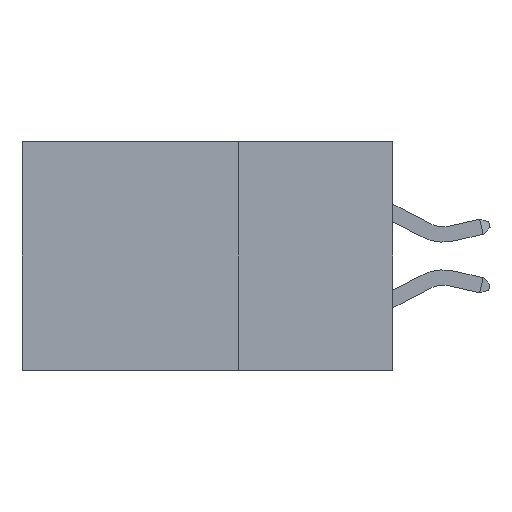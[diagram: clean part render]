
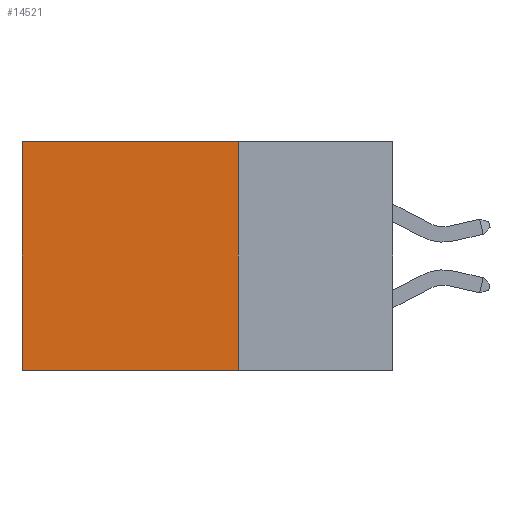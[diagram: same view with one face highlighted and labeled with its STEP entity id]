
A CAD part, left-side view. The second image highlights one B-rep face of the part: STEP entity #14521.
In plain terms, the highlighted planar face has unit normal (-1, 0, 0).
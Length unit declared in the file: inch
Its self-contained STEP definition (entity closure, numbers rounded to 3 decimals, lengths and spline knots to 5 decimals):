
#867 = EDGE_CURVE ( 'NONE', #17096, #4923, #8687, .T. ) ;
#1369 = ORIENTED_EDGE ( 'NONE', *, *, #20727, .F. ) ;
#3216 = ORIENTED_EDGE ( 'NONE', *, *, #12893, .T. ) ;
#4314 = LINE ( 'NONE', #5977, #14821 ) ;
#4923 = VERTEX_POINT ( 'NONE', #5642 ) ;
#5642 = CARTESIAN_POINT ( 'NONE',  ( 0.2875, 0.25, -0.37 ) ) ;
#5977 = CARTESIAN_POINT ( 'NONE',  ( 0.2875, 0.6, 0. ) ) ;
#6369 = CARTESIAN_POINT ( 'NONE',  ( 0.2875, 0.6, 0. ) ) ;
#6681 = VECTOR ( 'NONE', #17412, 39.37008 ) ;
#6877 = VECTOR ( 'NONE', #20412, 39.37008 ) ;
#6978 = VERTEX_POINT ( 'NONE', #6369 ) ;
#7198 = VERTEX_POINT ( 'NONE', #18804 ) ;
#7819 = AXIS2_PLACEMENT_3D ( 'NONE', #16612, #18407, #11796 ) ;
#8687 = LINE ( 'NONE', #13887, #6681 ) ;
#9073 = LINE ( 'NONE', #20928, #6877 ) ;
#9863 = EDGE_CURVE ( 'NONE', #17096, #6978, #9073, .T. ) ;
#11796 = DIRECTION ( 'NONE',  ( 0., 0., -1. ) ) ;
#12127 = ORIENTED_EDGE ( 'NONE', *, *, #9863, .T. ) ;
#12571 = CARTESIAN_POINT ( 'NONE',  ( 0.2875, 0.25, -0.37 ) ) ;
#12668 = LINE ( 'NONE', #12571, #19552 ) ;
#12893 = EDGE_CURVE ( 'NONE', #6978, #7198, #4314, .T. ) ;
#13887 = CARTESIAN_POINT ( 'NONE',  ( 0.2875, 0.25, 0. ) ) ;
#14521 = ADVANCED_FACE ( 'NONE', ( #14971 ), #20322, .F. ) ;
#14821 = VECTOR ( 'NONE', #17950, 39.37008 ) ;
#14971 = FACE_OUTER_BOUND ( 'NONE', #16584, .T. ) ;
#16584 = EDGE_LOOP ( 'NONE', ( #3216, #1369, #21742, #12127 ) ) ;
#16612 = CARTESIAN_POINT ( 'NONE',  ( 0.2875, 0.25, 0. ) ) ;
#17096 = VERTEX_POINT ( 'NONE', #19671 ) ;
#17412 = DIRECTION ( 'NONE',  ( 0., 0., -1. ) ) ;
#17950 = DIRECTION ( 'NONE',  ( 0., 0., -1. ) ) ;
#18407 = DIRECTION ( 'NONE',  ( 1., 0., 0. ) ) ;
#18804 = CARTESIAN_POINT ( 'NONE',  ( 0.2875, 0.6, -0.37 ) ) ;
#19552 = VECTOR ( 'NONE', #21405, 39.37008 ) ;
#19671 = CARTESIAN_POINT ( 'NONE',  ( 0.2875, 0.25, 0. ) ) ;
#20322 = PLANE ( 'NONE',  #7819 ) ;
#20412 = DIRECTION ( 'NONE',  ( 0., 1., 0. ) ) ;
#20727 = EDGE_CURVE ( 'NONE', #4923, #7198, #12668, .T. ) ;
#20928 = CARTESIAN_POINT ( 'NONE',  ( 0.2875, 0.25, 0. ) ) ;
#21405 = DIRECTION ( 'NONE',  ( 0., 1., 0. ) ) ;
#21742 = ORIENTED_EDGE ( 'NONE', *, *, #867, .F. ) ;
